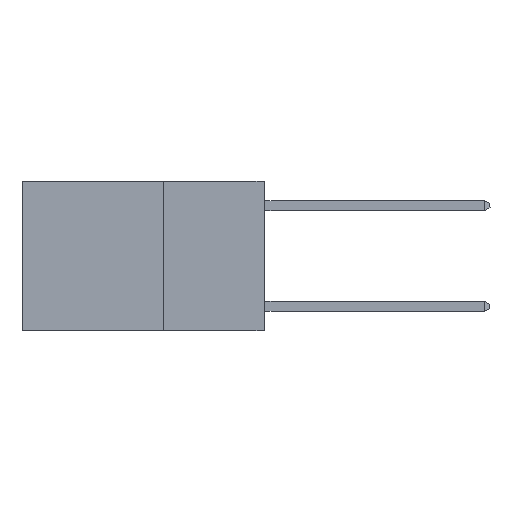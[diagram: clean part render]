
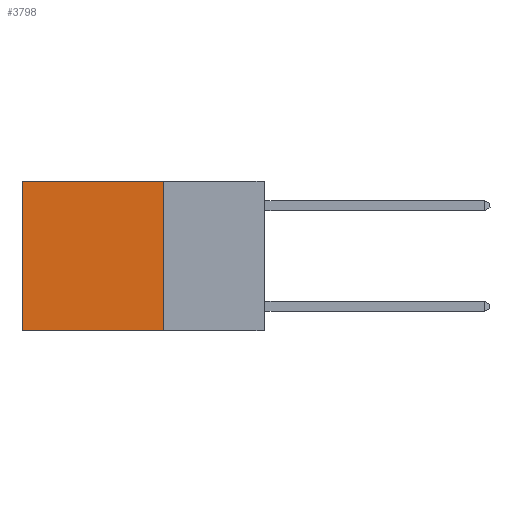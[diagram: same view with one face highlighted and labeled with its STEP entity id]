
A CAD part, left-side view. The second image highlights one B-rep face of the part: STEP entity #3798.
In plain terms, the highlighted planar face has unit normal (-1, 0, 0).
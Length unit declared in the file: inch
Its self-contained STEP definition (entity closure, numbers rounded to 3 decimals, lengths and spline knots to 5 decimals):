
#24 = CARTESIAN_POINT ( 'NONE',  ( 0.2625, 0.6, 0. ) ) ;
#349 = VERTEX_POINT ( 'NONE', #7018 ) ;
#680 = VERTEX_POINT ( 'NONE', #6270 ) ;
#1034 = EDGE_CURVE ( 'NONE', #5197, #349, #5659, .T. ) ;
#1494 = VECTOR ( 'NONE', #5303, 39.37008 ) ;
#1739 = EDGE_LOOP ( 'NONE', ( #5493, #4571, #6259, #6400 ) ) ;
#1850 = DIRECTION ( 'NONE',  ( 1., 0., 0. ) ) ;
#1865 = DIRECTION ( 'NONE',  ( 0., 1., 0. ) ) ;
#2373 = VECTOR ( 'NONE', #9064, 39.37008 ) ;
#2630 = CARTESIAN_POINT ( 'NONE',  ( 0.2625, 0.25, 0. ) ) ;
#3196 = CARTESIAN_POINT ( 'NONE',  ( 0.2625, 0.25, -0.37 ) ) ;
#3387 = EDGE_CURVE ( 'NONE', #349, #680, #9986, .T. ) ;
#3798 = ADVANCED_FACE ( 'NONE', ( #7564 ), #7742, .F. ) ;
#4208 = CARTESIAN_POINT ( 'NONE',  ( 0.2625, 0.25, 0. ) ) ;
#4445 = DIRECTION ( 'NONE',  ( 0., 0., -1. ) ) ;
#4464 = VECTOR ( 'NONE', #1865, 39.37008 ) ;
#4571 = ORIENTED_EDGE ( 'NONE', *, *, #9588, .F. ) ;
#5093 = LINE ( 'NONE', #9956, #8573 ) ;
#5197 = VERTEX_POINT ( 'NONE', #4208 ) ;
#5303 = DIRECTION ( 'NONE',  ( 0., 0., -1. ) ) ;
#5493 = ORIENTED_EDGE ( 'NONE', *, *, #3387, .T. ) ;
#5659 = LINE ( 'NONE', #2630, #4464 ) ;
#5881 = LINE ( 'NONE', #3196, #2373 ) ;
#6259 = ORIENTED_EDGE ( 'NONE', *, *, #9651, .F. ) ;
#6270 = CARTESIAN_POINT ( 'NONE',  ( 0.2625, 0.6, -0.37 ) ) ;
#6400 = ORIENTED_EDGE ( 'NONE', *, *, #1034, .T. ) ;
#7018 = CARTESIAN_POINT ( 'NONE',  ( 0.2625, 0.6, 0. ) ) ;
#7179 = VERTEX_POINT ( 'NONE', #8925 ) ;
#7518 = AXIS2_PLACEMENT_3D ( 'NONE', #8344, #1850, #4445 ) ;
#7564 = FACE_OUTER_BOUND ( 'NONE', #1739, .T. ) ;
#7742 = PLANE ( 'NONE',  #7518 ) ;
#8344 = CARTESIAN_POINT ( 'NONE',  ( 0.2625, 0.25, 0. ) ) ;
#8573 = VECTOR ( 'NONE', #9174, 39.37008 ) ;
#8925 = CARTESIAN_POINT ( 'NONE',  ( 0.2625, 0.25, -0.37 ) ) ;
#9064 = DIRECTION ( 'NONE',  ( 0., 1., 0. ) ) ;
#9174 = DIRECTION ( 'NONE',  ( 0., 0., -1. ) ) ;
#9588 = EDGE_CURVE ( 'NONE', #7179, #680, #5881, .T. ) ;
#9651 = EDGE_CURVE ( 'NONE', #5197, #7179, #5093, .T. ) ;
#9956 = CARTESIAN_POINT ( 'NONE',  ( 0.2625, 0.25, 0. ) ) ;
#9986 = LINE ( 'NONE', #24, #1494 ) ;
